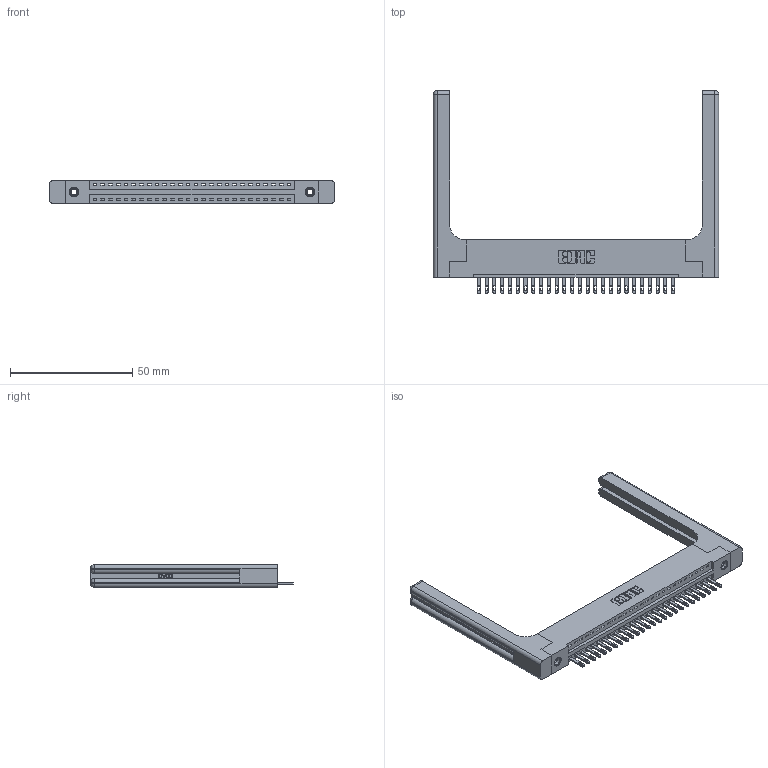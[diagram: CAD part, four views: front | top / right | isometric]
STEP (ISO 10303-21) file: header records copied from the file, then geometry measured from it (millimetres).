
FILE_DESCRIPTION (( 'STEP AP203' ), '1' );
FILE_NAME ('346-026-500-158.STEP', '2022-05-06T01:51:22', ( '' ), ( '' ), 'SwSTEP 2.0', 'SolidWorks 2020', '' );
FILE_SCHEMA (( 'CONFIG_CONTROL_DESIGN' ));
Length unit declared in the file: inch
Products named in the file (5): 346-220-058_345-220-058; 345-250-001_345-250-001-102; 346 Part_Flush Mounting Lugs - 0.156 Dia-TH; 346-026-500-158; 345-292-001_345-293-100
Assembly tree (31 placements, depth 2):
  346-026-500-158
    346 Part_Flush Mounting Lugs - 0.156 Dia-TH
    345-292-001_345-293-100  x26
    345-250-001_345-250-001-102  x2
    346-220-058_345-220-058  x2
Bounding box: 116.61 x 82.8 x 9.4 mm (x, y, z)
Volume: 18568.4 mm3; surface area: 18900.9 mm2
Topology: 31 solids, 31 shells, 1796 faces, 5399 edges, 3578 vertices
Faces by surface type: plane 1122, cylinder 614, bspline 36, cone 12, sphere 8, torus 4
Entity records: 23818 total; most frequent: CARTESIAN_POINT 5069, ORIENTED_EDGE 3824, DIRECTION 3424, EDGE_CURVE 1912, VECTOR 1580, LINE 1580, VERTEX_POINT 1266, AXIS2_PLACEMENT_3D 922
